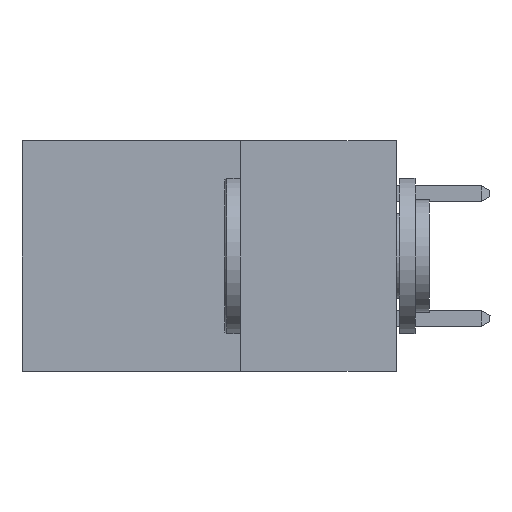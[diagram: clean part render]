
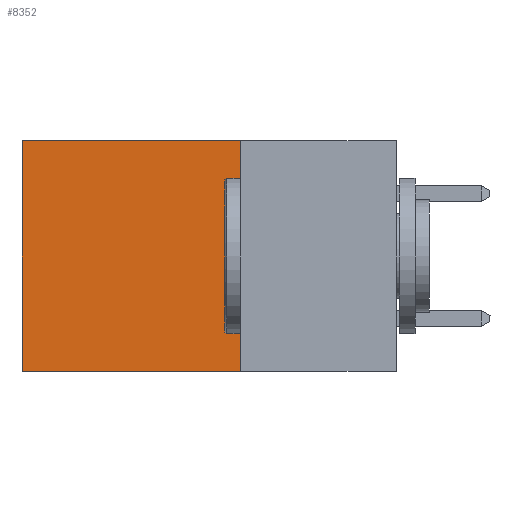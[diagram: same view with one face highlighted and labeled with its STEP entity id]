
A CAD part, left-side view. The second image highlights one B-rep face of the part: STEP entity #8352.
In plain terms, the highlighted planar face has unit normal (-1, 0, 0).
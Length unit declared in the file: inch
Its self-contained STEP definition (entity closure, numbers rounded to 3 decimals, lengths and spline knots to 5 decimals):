
#177 = LINE ( 'NONE', #5706, #2134 ) ;
#478 = ORIENTED_EDGE ( 'NONE', *, *, #1258, .F. ) ;
#1189 = CARTESIAN_POINT ( 'NONE',  ( 0.2615, 0.25, -0.37 ) ) ;
#1258 = EDGE_CURVE ( 'NONE', #2347, #3503, #2609, .T. ) ;
#1517 = AXIS2_PLACEMENT_3D ( 'NONE', #1189, #7310, #2008 ) ;
#1655 = CARTESIAN_POINT ( 'NONE',  ( 0.2615, 0.6, -0.37 ) ) ;
#1695 = LINE ( 'NONE', #7994, #5830 ) ;
#1933 = CARTESIAN_POINT ( 'NONE',  ( 0.2615, 0.25, -0.37 ) ) ;
#2008 = DIRECTION ( 'NONE',  ( 0., 0., -1. ) ) ;
#2134 = VECTOR ( 'NONE', #5691, 39.37008 ) ;
#2347 = VERTEX_POINT ( 'NONE', #4562 ) ;
#2411 = CARTESIAN_POINT ( 'NONE',  ( 0.2615, 0.25, -0.37 ) ) ;
#2609 = LINE ( 'NONE', #1933, #9602 ) ;
#2768 = ORIENTED_EDGE ( 'NONE', *, *, #4478, .T. ) ;
#3503 = VERTEX_POINT ( 'NONE', #2411 ) ;
#4478 = EDGE_CURVE ( 'NONE', #9036, #5071, #177, .T. ) ;
#4562 = CARTESIAN_POINT ( 'NONE',  ( 0.2615, 0.25, 0. ) ) ;
#5071 = VERTEX_POINT ( 'NONE', #1655 ) ;
#5126 = LINE ( 'NONE', #7816, #9500 ) ;
#5513 = PLANE ( 'NONE',  #1517 ) ;
#5691 = DIRECTION ( 'NONE',  ( 0., 0., -1. ) ) ;
#5706 = CARTESIAN_POINT ( 'NONE',  ( 0.2615, 0.6, -0.37 ) ) ;
#5830 = VECTOR ( 'NONE', #8856, 39.37008 ) ;
#6015 = FACE_OUTER_BOUND ( 'NONE', #6355, .T. ) ;
#6355 = EDGE_LOOP ( 'NONE', ( #2768, #7870, #478, #8299 ) ) ;
#7310 = DIRECTION ( 'NONE',  ( 1., 0., 0. ) ) ;
#7816 = CARTESIAN_POINT ( 'NONE',  ( 0.2615, 0.25, -0.37 ) ) ;
#7870 = ORIENTED_EDGE ( 'NONE', *, *, #10992, .F. ) ;
#7994 = CARTESIAN_POINT ( 'NONE',  ( 0.2615, 0.25, 0. ) ) ;
#8299 = ORIENTED_EDGE ( 'NONE', *, *, #11118, .T. ) ;
#8352 = ADVANCED_FACE ( 'NONE', ( #6015 ), #5513, .F. ) ;
#8556 = CARTESIAN_POINT ( 'NONE',  ( 0.2615, 0.6, 0. ) ) ;
#8856 = DIRECTION ( 'NONE',  ( 0., 1., 0. ) ) ;
#9036 = VERTEX_POINT ( 'NONE', #8556 ) ;
#9500 = VECTOR ( 'NONE', #11261, 39.37008 ) ;
#9602 = VECTOR ( 'NONE', #10224, 39.37008 ) ;
#10224 = DIRECTION ( 'NONE',  ( 0., 0., -1. ) ) ;
#10992 = EDGE_CURVE ( 'NONE', #3503, #5071, #5126, .T. ) ;
#11118 = EDGE_CURVE ( 'NONE', #2347, #9036, #1695, .T. ) ;
#11261 = DIRECTION ( 'NONE',  ( 0., 1., 0. ) ) ;
